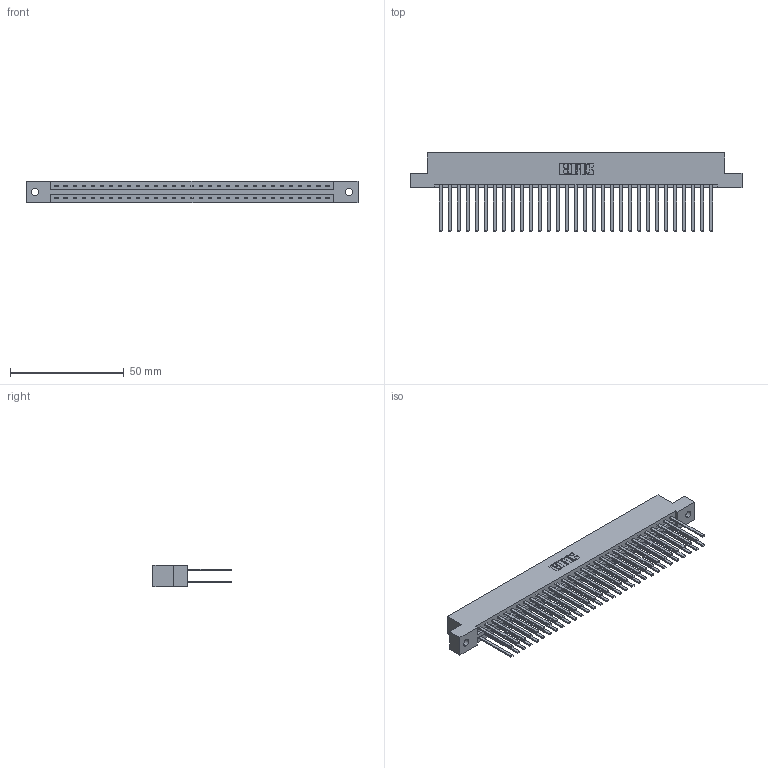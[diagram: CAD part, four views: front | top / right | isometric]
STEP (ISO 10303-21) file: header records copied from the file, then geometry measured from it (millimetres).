
FILE_DESCRIPTION (( 'STEP AP203' ), '1' );
FILE_NAME ('337-062-544-202.STEP', '2019-10-09T21:27:46', ( '' ), ( '' ), 'SwSTEP 2.0', 'SolidWorks 2016', '' );
FILE_SCHEMA (( 'CONFIG_CONTROL_DESIGN' ));
Length unit declared in the file: inch
Products named in the file (3): 337 Part_Flush Mounting Lugs - 0.128 Dia; 345-292-001_345-293-144; 337-062-544-202
Assembly tree (63 placements, depth 2):
  337-062-544-202
    337 Part_Flush Mounting Lugs - 0.128 Dia
    345-292-001_345-293-144  x62
Bounding box: 145.85 x 34.3 x 9.4 mm (x, y, z)
Volume: 16056.5 mm3; surface area: 20611.6 mm2
Topology: 63 solids, 63 shells, 3090 faces, 9177 edges, 6034 vertices
Faces by surface type: plane 2178, cylinder 912
Entity records: 25277 total; most frequent: CARTESIAN_POINT 4266, ORIENTED_EDGE 4202, DIRECTION 3645, EDGE_CURVE 2101, LINE 1977, VECTOR 1977, VERTEX_POINT 1398, AXIS2_PLACEMENT_3D 834
